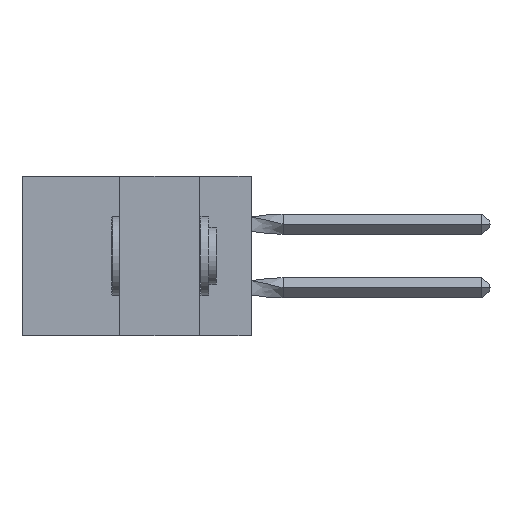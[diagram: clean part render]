
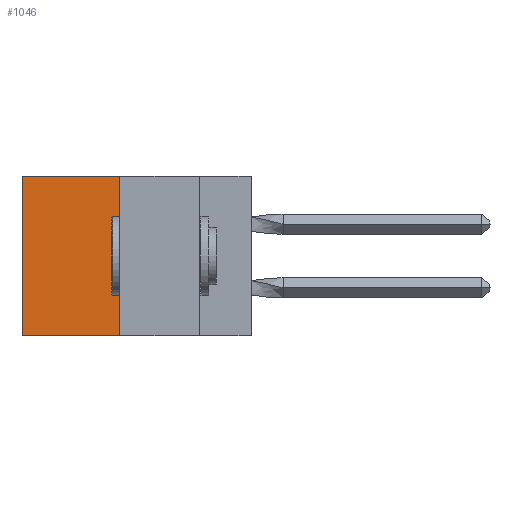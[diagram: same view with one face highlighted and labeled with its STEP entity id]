
A CAD part, left-side view. The second image highlights one B-rep face of the part: STEP entity #1046.
In plain terms, the highlighted planar face has unit normal (-1, 0, 0).
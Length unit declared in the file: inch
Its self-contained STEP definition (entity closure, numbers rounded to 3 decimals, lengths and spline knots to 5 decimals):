
#824 = EDGE_CURVE ( 'NONE', #1223, #20915, #8618, .T. ) ;
#919 = DIRECTION ( 'NONE',  ( 1., 0., 0. ) ) ;
#945 = VECTOR ( 'NONE', #5603, 39.37008 ) ;
#1046 = ADVANCED_FACE ( 'NONE', ( #23343 ), #8211, .F. ) ;
#1223 = VERTEX_POINT ( 'NONE', #13086 ) ;
#1301 = CARTESIAN_POINT ( 'NONE',  ( 0.305, 0.413, -0.5 ) ) ;
#1488 = ORIENTED_EDGE ( 'NONE', *, *, #17903, .F. ) ;
#1767 = CARTESIAN_POINT ( 'NONE',  ( 0.305, 0.413, 0. ) ) ;
#2611 = EDGE_CURVE ( 'NONE', #13033, #20915, #8007, .T. ) ;
#5161 = VECTOR ( 'NONE', #22802, 39.37008 ) ;
#5603 = DIRECTION ( 'NONE',  ( 0., 0., -1. ) ) ;
#6375 = EDGE_LOOP ( 'NONE', ( #12386, #16512, #1488, #16102 ) ) ;
#8007 = LINE ( 'NONE', #8299, #5161 ) ;
#8211 = PLANE ( 'NONE',  #10324 ) ;
#8299 = CARTESIAN_POINT ( 'NONE',  ( 0.305, 0.413, -0.5 ) ) ;
#8618 = LINE ( 'NONE', #22401, #22524 ) ;
#10087 = EDGE_CURVE ( 'NONE', #18151, #1223, #13641, .T. ) ;
#10324 = AXIS2_PLACEMENT_3D ( 'NONE', #1301, #919, #22637 ) ;
#10631 = DIRECTION ( 'NONE',  ( 0., 1., 0. ) ) ;
#10708 = CARTESIAN_POINT ( 'NONE',  ( 0.305, 0.413, 0. ) ) ;
#12386 = ORIENTED_EDGE ( 'NONE', *, *, #824, .T. ) ;
#12594 = CARTESIAN_POINT ( 'NONE',  ( 0.305, 0.413, -0.5 ) ) ;
#13033 = VERTEX_POINT ( 'NONE', #12594 ) ;
#13086 = CARTESIAN_POINT ( 'NONE',  ( 0.305, 0.72, 0. ) ) ;
#13641 = LINE ( 'NONE', #1767, #17342 ) ;
#16102 = ORIENTED_EDGE ( 'NONE', *, *, #10087, .T. ) ;
#16512 = ORIENTED_EDGE ( 'NONE', *, *, #2611, .F. ) ;
#17342 = VECTOR ( 'NONE', #10631, 39.37008 ) ;
#17903 = EDGE_CURVE ( 'NONE', #18151, #13033, #17948, .T. ) ;
#17948 = LINE ( 'NONE', #19590, #945 ) ;
#18151 = VERTEX_POINT ( 'NONE', #10708 ) ;
#19590 = CARTESIAN_POINT ( 'NONE',  ( 0.305, 0.413, -0.5 ) ) ;
#20692 = DIRECTION ( 'NONE',  ( 0., 0., -1. ) ) ;
#20915 = VERTEX_POINT ( 'NONE', #22672 ) ;
#22401 = CARTESIAN_POINT ( 'NONE',  ( 0.305, 0.72, -0.5 ) ) ;
#22524 = VECTOR ( 'NONE', #20692, 39.37008 ) ;
#22637 = DIRECTION ( 'NONE',  ( 0., 0., -1. ) ) ;
#22672 = CARTESIAN_POINT ( 'NONE',  ( 0.305, 0.72, -0.5 ) ) ;
#22802 = DIRECTION ( 'NONE',  ( 0., 1., 0. ) ) ;
#23343 = FACE_OUTER_BOUND ( 'NONE', #6375, .T. ) ;
